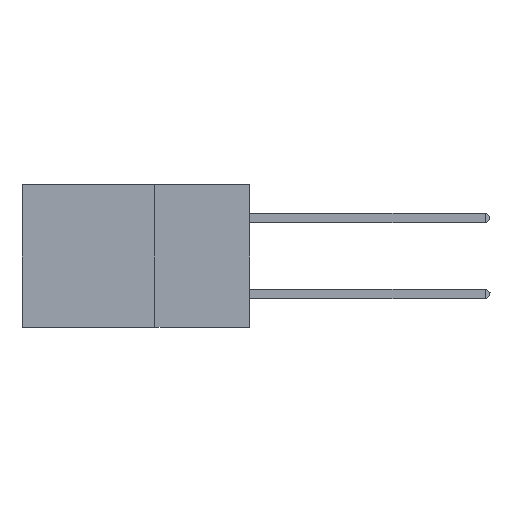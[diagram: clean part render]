
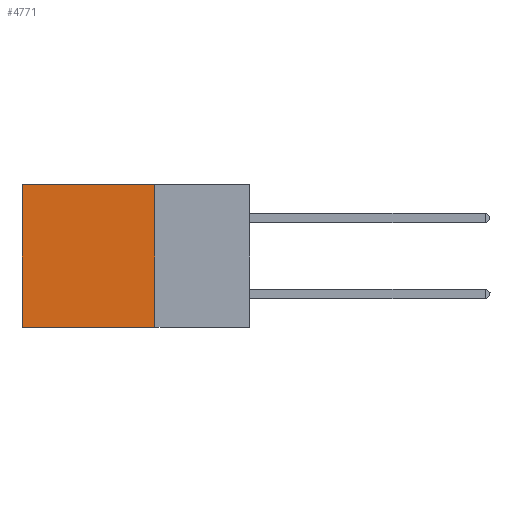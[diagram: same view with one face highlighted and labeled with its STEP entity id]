
A CAD part, left-side view. The second image highlights one B-rep face of the part: STEP entity #4771.
In plain terms, the highlighted planar face has unit normal (-1, 0, 0).
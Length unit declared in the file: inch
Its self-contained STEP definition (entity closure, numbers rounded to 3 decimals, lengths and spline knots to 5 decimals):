
#758 = DIRECTION ( 'NONE',  ( 0., 1., 0. ) ) ;
#1248 = CARTESIAN_POINT ( 'NONE',  ( 0.2875, 0.25, -0.375 ) ) ;
#1605 = CARTESIAN_POINT ( 'NONE',  ( 0.2875, 0.6, -0.375 ) ) ;
#2039 = LINE ( 'NONE', #3538, #13182 ) ;
#2955 = CARTESIAN_POINT ( 'NONE',  ( 0.2875, 0.25, 0. ) ) ;
#3414 = ORIENTED_EDGE ( 'NONE', *, *, #15517, .T. ) ;
#3538 = CARTESIAN_POINT ( 'NONE',  ( 0.2875, 0.25, -0.375 ) ) ;
#4295 = EDGE_CURVE ( 'NONE', #15636, #9872, #2039, .T. ) ;
#4771 = ADVANCED_FACE ( 'NONE', ( #10637 ), #12029, .F. ) ;
#5260 = ORIENTED_EDGE ( 'NONE', *, *, #6323, .T. ) ;
#5599 = AXIS2_PLACEMENT_3D ( 'NONE', #17769, #11826, #6070 ) ;
#6070 = DIRECTION ( 'NONE',  ( 0., 0., -1. ) ) ;
#6323 = EDGE_CURVE ( 'NONE', #17666, #8172, #11488, .T. ) ;
#7181 = VECTOR ( 'NONE', #16217, 39.37008 ) ;
#7426 = CARTESIAN_POINT ( 'NONE',  ( 0.2875, 0.6, -0.375 ) ) ;
#8172 = VERTEX_POINT ( 'NONE', #7426 ) ;
#9129 = DIRECTION ( 'NONE',  ( 0., 0., -1. ) ) ;
#9872 = VERTEX_POINT ( 'NONE', #1248 ) ;
#10637 = FACE_OUTER_BOUND ( 'NONE', #12462, .T. ) ;
#11488 = LINE ( 'NONE', #1605, #7181 ) ;
#11826 = DIRECTION ( 'NONE',  ( 1., 0., 0. ) ) ;
#12029 = PLANE ( 'NONE',  #5599 ) ;
#12274 = VECTOR ( 'NONE', #14732, 39.37008 ) ;
#12462 = EDGE_LOOP ( 'NONE', ( #5260, #15841, #16097, #3414 ) ) ;
#12963 = CARTESIAN_POINT ( 'NONE',  ( 0.2875, 0.6, 0. ) ) ;
#13182 = VECTOR ( 'NONE', #9129, 39.37008 ) ;
#14732 = DIRECTION ( 'NONE',  ( 0., 1., 0. ) ) ;
#15081 = EDGE_CURVE ( 'NONE', #9872, #8172, #17274, .T. ) ;
#15312 = CARTESIAN_POINT ( 'NONE',  ( 0.2875, 0.25, -0.375 ) ) ;
#15517 = EDGE_CURVE ( 'NONE', #15636, #17666, #16588, .T. ) ;
#15636 = VERTEX_POINT ( 'NONE', #16316 ) ;
#15841 = ORIENTED_EDGE ( 'NONE', *, *, #15081, .F. ) ;
#16097 = ORIENTED_EDGE ( 'NONE', *, *, #4295, .F. ) ;
#16217 = DIRECTION ( 'NONE',  ( 0., 0., -1. ) ) ;
#16316 = CARTESIAN_POINT ( 'NONE',  ( 0.2875, 0.25, 0. ) ) ;
#16588 = LINE ( 'NONE', #2955, #12274 ) ;
#17274 = LINE ( 'NONE', #15312, #18670 ) ;
#17666 = VERTEX_POINT ( 'NONE', #12963 ) ;
#17769 = CARTESIAN_POINT ( 'NONE',  ( 0.2875, 0.25, -0.375 ) ) ;
#18670 = VECTOR ( 'NONE', #758, 39.37008 ) ;
